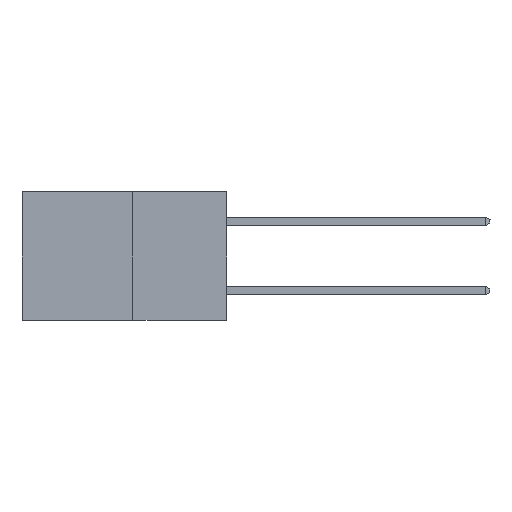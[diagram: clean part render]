
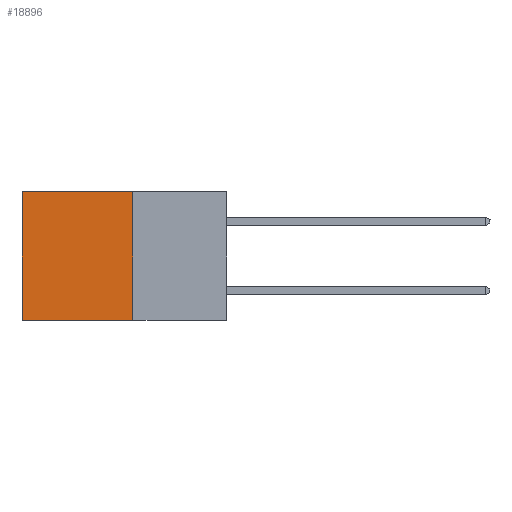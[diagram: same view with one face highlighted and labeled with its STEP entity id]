
A CAD part, left-side view. The second image highlights one B-rep face of the part: STEP entity #18896.
In plain terms, the highlighted planar face has unit normal (-1, 0, 0).
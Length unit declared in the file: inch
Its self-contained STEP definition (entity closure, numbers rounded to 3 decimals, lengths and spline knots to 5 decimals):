
#7 = LINE ( 'NONE', #9972, #1793 ) ;
#628 = DIRECTION ( 'NONE',  ( 0., 1., 0. ) ) ;
#695 = CARTESIAN_POINT ( 'NONE',  ( 0.277, 0.27, -0.37 ) ) ;
#751 = VECTOR ( 'NONE', #16139, 39.37008 ) ;
#1529 = DIRECTION ( 'NONE',  ( 0., 0., -1. ) ) ;
#1793 = VECTOR ( 'NONE', #15676, 39.37008 ) ;
#2490 = CARTESIAN_POINT ( 'NONE',  ( 0.277, 0.59, 0. ) ) ;
#2587 = DIRECTION ( 'NONE',  ( 1., 0., 0. ) ) ;
#4387 = FACE_OUTER_BOUND ( 'NONE', #11531, .T. ) ;
#5389 = EDGE_CURVE ( 'NONE', #23219, #10213, #15042, .T. ) ;
#6307 = VERTEX_POINT ( 'NONE', #2490 ) ;
#6701 = CARTESIAN_POINT ( 'NONE',  ( 0.277, 0.27, 0. ) ) ;
#7977 = CARTESIAN_POINT ( 'NONE',  ( 0.277, 0.27, -0.37 ) ) ;
#9030 = EDGE_CURVE ( 'NONE', #10213, #9579, #14467, .T. ) ;
#9579 = VERTEX_POINT ( 'NONE', #19428 ) ;
#9972 = CARTESIAN_POINT ( 'NONE',  ( 0.277, 0.27, 0. ) ) ;
#10031 = VECTOR ( 'NONE', #1529, 39.37008 ) ;
#10213 = VERTEX_POINT ( 'NONE', #7977 ) ;
#11165 = ORIENTED_EDGE ( 'NONE', *, *, #9030, .F. ) ;
#11196 = AXIS2_PLACEMENT_3D ( 'NONE', #695, #2587, #15862 ) ;
#11531 = EDGE_LOOP ( 'NONE', ( #21445, #11165, #12862, #12016 ) ) ;
#12016 = ORIENTED_EDGE ( 'NONE', *, *, #13233, .T. ) ;
#12862 = ORIENTED_EDGE ( 'NONE', *, *, #5389, .F. ) ;
#13233 = EDGE_CURVE ( 'NONE', #23219, #6307, #7, .T. ) ;
#13946 = PLANE ( 'NONE',  #11196 ) ;
#14065 = EDGE_CURVE ( 'NONE', #6307, #9579, #16459, .T. ) ;
#14214 = CARTESIAN_POINT ( 'NONE',  ( 0.277, 0.59, -0.37 ) ) ;
#14467 = LINE ( 'NONE', #23342, #23956 ) ;
#14783 = CARTESIAN_POINT ( 'NONE',  ( 0.277, 0.27, -0.37 ) ) ;
#15042 = LINE ( 'NONE', #14783, #10031 ) ;
#15676 = DIRECTION ( 'NONE',  ( 0., 1., 0. ) ) ;
#15862 = DIRECTION ( 'NONE',  ( 0., 0., -1. ) ) ;
#16139 = DIRECTION ( 'NONE',  ( 0., 0., -1. ) ) ;
#16459 = LINE ( 'NONE', #14214, #751 ) ;
#18896 = ADVANCED_FACE ( 'NONE', ( #4387 ), #13946, .F. ) ;
#19428 = CARTESIAN_POINT ( 'NONE',  ( 0.277, 0.59, -0.37 ) ) ;
#21445 = ORIENTED_EDGE ( 'NONE', *, *, #14065, .T. ) ;
#23219 = VERTEX_POINT ( 'NONE', #6701 ) ;
#23342 = CARTESIAN_POINT ( 'NONE',  ( 0.277, 0.27, -0.37 ) ) ;
#23956 = VECTOR ( 'NONE', #628, 39.37008 ) ;
